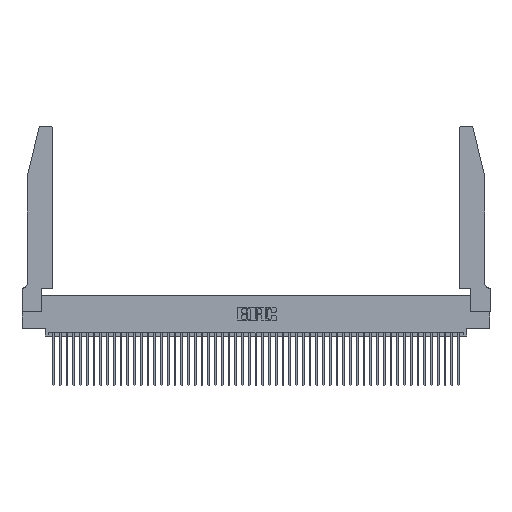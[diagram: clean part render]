
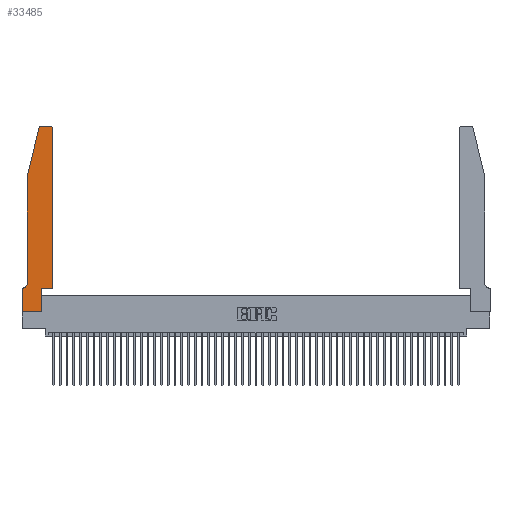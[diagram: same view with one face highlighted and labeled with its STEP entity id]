
A CAD part, top view. The second image highlights one B-rep face of the part: STEP entity #33485.
In plain terms, the highlighted planar face has unit normal (0, 0, 1).
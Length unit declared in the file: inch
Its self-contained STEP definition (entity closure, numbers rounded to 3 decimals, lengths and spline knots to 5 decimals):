
#647 = ORIENTED_EDGE ( 'NONE', *, *, #27246, .T. ) ;
#713 = LINE ( 'NONE', #17386, #20215 ) ;
#718 = CARTESIAN_POINT ( 'NONE',  ( 0.4505, 2.72, 0.37 ) ) ;
#2544 = EDGE_CURVE ( 'NONE', #25162, #24397, #713, .T. ) ;
#3590 = CARTESIAN_POINT ( 'NONE',  ( 0.0755, 2., 0.37 ) ) ;
#3707 = CARTESIAN_POINT ( 'NONE',  ( 0.2865, 0.35, 0.37 ) ) ;
#4420 = VECTOR ( 'NONE', #8207, 39.37008 ) ;
#6804 = ORIENTED_EDGE ( 'NONE', *, *, #12486, .T. ) ;
#7008 = DIRECTION ( 'NONE',  ( 0., 0., 1. ) ) ;
#7014 = DIRECTION ( 'NONE',  ( 0., 0., 1. ) ) ;
#7087 = VERTEX_POINT ( 'NONE', #14316 ) ;
#7631 = EDGE_LOOP ( 'NONE', ( #6804, #647, #19956, #20746, #41862, #13856, #21926, #33916, #32692, #13789, #16036, #45200 ) ) ;
#7732 = AXIS2_PLACEMENT_3D ( 'NONE', #43653, #20434, #47519 ) ;
#7896 = DIRECTION ( 'NONE',  ( 1., 0., 0. ) ) ;
#8207 = DIRECTION ( 'NONE',  ( -1., 0., 0. ) ) ;
#8855 = AXIS2_PLACEMENT_3D ( 'NONE', #42272, #19062, #46180 ) ;
#10037 = VERTEX_POINT ( 'NONE', #38490 ) ;
#12369 = VERTEX_POINT ( 'NONE', #46196 ) ;
#12486 = EDGE_CURVE ( 'NONE', #16111, #10037, #36589, .T. ) ;
#12656 = VECTOR ( 'NONE', #7896, 39.37008 ) ;
#12976 = EDGE_CURVE ( 'NONE', #24397, #7087, #18510, .T. ) ;
#13789 = ORIENTED_EDGE ( 'NONE', *, *, #38945, .T. ) ;
#13843 = DIRECTION ( 'NONE',  ( -1., 0., 0. ) ) ;
#13856 = ORIENTED_EDGE ( 'NONE', *, *, #46249, .T. ) ;
#13866 = LINE ( 'NONE', #15563, #12656 ) ;
#14316 = CARTESIAN_POINT ( 'NONE',  ( 0.2865, 0.35, 0.37 ) ) ;
#15222 = PLANE ( 'NONE',  #8855 ) ;
#15262 = CARTESIAN_POINT ( 'NONE',  ( 0.4505, 0.35, 0.37 ) ) ;
#15388 = CARTESIAN_POINT ( 'NONE',  ( 0., 0., 0.37 ) ) ;
#15453 = EDGE_CURVE ( 'NONE', #23237, #16111, #32829, .T. ) ;
#15563 = CARTESIAN_POINT ( 'NONE',  ( 0.4505, 0.35, 0.37 ) ) ;
#15775 = CARTESIAN_POINT ( 'NONE',  ( 0.25487, 2.72718, 0.37 ) ) ;
#16036 = ORIENTED_EDGE ( 'NONE', *, *, #18332, .T. ) ;
#16111 = VERTEX_POINT ( 'NONE', #19169 ) ;
#17232 = DIRECTION ( 'NONE',  ( 0., -1., 0. ) ) ;
#17386 = CARTESIAN_POINT ( 'NONE',  ( 0., 0., 0.37 ) ) ;
#17463 = VERTEX_POINT ( 'NONE', #41365 ) ;
#18332 = EDGE_CURVE ( 'NONE', #20852, #23237, #23528, .T. ) ;
#18510 = LINE ( 'NONE', #3707, #48184 ) ;
#19062 = DIRECTION ( 'NONE',  ( 0., 0., 1. ) ) ;
#19169 = CARTESIAN_POINT ( 'NONE',  ( 0.4205, 2.75, 0.37 ) ) ;
#19956 = ORIENTED_EDGE ( 'NONE', *, *, #48981, .T. ) ;
#20215 = VECTOR ( 'NONE', #44496, 39.37008 ) ;
#20434 = DIRECTION ( 'NONE',  ( 0., 0., -1. ) ) ;
#20746 = ORIENTED_EDGE ( 'NONE', *, *, #31628, .T. ) ;
#20852 = VERTEX_POINT ( 'NONE', #49442 ) ;
#21926 = ORIENTED_EDGE ( 'NONE', *, *, #24889, .T. ) ;
#23237 = VERTEX_POINT ( 'NONE', #718 ) ;
#23528 = LINE ( 'NONE', #15262, #44100 ) ;
#24397 = VERTEX_POINT ( 'NONE', #30204 ) ;
#24889 = EDGE_CURVE ( 'NONE', #26045, #25162, #47878, .T. ) ;
#25162 = VERTEX_POINT ( 'NONE', #15388 ) ;
#25265 = VECTOR ( 'NONE', #39976, 39.37008 ) ;
#26044 = LINE ( 'NONE', #3590, #33894 ) ;
#26045 = VERTEX_POINT ( 'NONE', #29202 ) ;
#26130 = VECTOR ( 'NONE', #17232, 39.37008 ) ;
#26546 = CIRCLE ( 'NONE', #36885, 0.03 ) ;
#27246 = EDGE_CURVE ( 'NONE', #10037, #40336, #26546, .T. ) ;
#28882 = VERTEX_POINT ( 'NONE', #28950 ) ;
#28950 = CARTESIAN_POINT ( 'NONE',  ( 0.0755, 2., 0.37 ) ) ;
#29202 = CARTESIAN_POINT ( 'NONE',  ( 0., 0.35, 0.37 ) ) ;
#29277 = CARTESIAN_POINT ( 'NONE',  ( 0.0755, 0.35, 0.37 ) ) ;
#30204 = CARTESIAN_POINT ( 'NONE',  ( 0.2865, 0., 0.37 ) ) ;
#30283 = CARTESIAN_POINT ( 'NONE',  ( 0.4205, 2.72, 0.37 ) ) ;
#30292 = CARTESIAN_POINT ( 'NONE',  ( 0.284, 2.72, 0.37 ) ) ;
#30936 = LINE ( 'NONE', #29277, #46584 ) ;
#31628 = EDGE_CURVE ( 'NONE', #28882, #17463, #26044, .T. ) ;
#32218 = CARTESIAN_POINT ( 'NONE',  ( 0.0755, 2., 0.37 ) ) ;
#32692 = ORIENTED_EDGE ( 'NONE', *, *, #12976, .T. ) ;
#32829 = CIRCLE ( 'NONE', #35489, 0.03 ) ;
#33485 = ADVANCED_FACE ( 'NONE', ( #45192 ), #15222, .T. ) ;
#33894 = VECTOR ( 'NONE', #50013, 39.37008 ) ;
#33916 = ORIENTED_EDGE ( 'NONE', *, *, #2544, .T. ) ;
#34160 = DIRECTION ( 'NONE',  ( 1., 0., 0. ) ) ;
#34165 = DIRECTION ( 'NONE',  ( 1., 0., 0. ) ) ;
#34785 = DIRECTION ( 'NONE',  ( 0., 1., 0. ) ) ;
#35314 = CARTESIAN_POINT ( 'NONE',  ( 0.2605, 2.75, 0.37 ) ) ;
#35489 = AXIS2_PLACEMENT_3D ( 'NONE', #30283, #7008, #34160 ) ;
#35512 = LINE ( 'NONE', #32218, #25265 ) ;
#36040 = CIRCLE ( 'NONE', #7732, 0.07 ) ;
#36589 = LINE ( 'NONE', #35314, #4420 ) ;
#36885 = AXIS2_PLACEMENT_3D ( 'NONE', #30292, #7014, #34165 ) ;
#38411 = DIRECTION ( 'NONE',  ( 0., 1., 0. ) ) ;
#38490 = CARTESIAN_POINT ( 'NONE',  ( 0.284, 2.75, 0.37 ) ) ;
#38945 = EDGE_CURVE ( 'NONE', #7087, #20852, #13866, .T. ) ;
#39976 = DIRECTION ( 'NONE',  ( -0.239, -0.971, 0. ) ) ;
#40336 = VERTEX_POINT ( 'NONE', #15775 ) ;
#40891 = EDGE_CURVE ( 'NONE', #17463, #12369, #36040, .T. ) ;
#41365 = CARTESIAN_POINT ( 'NONE',  ( 0.0755, 0.42, 0.37 ) ) ;
#41862 = ORIENTED_EDGE ( 'NONE', *, *, #40891, .T. ) ;
#42272 = CARTESIAN_POINT ( 'NONE',  ( 0., 0.35, 0.37 ) ) ;
#43653 = CARTESIAN_POINT ( 'NONE',  ( 0.0055, 0.42, 0.37 ) ) ;
#44100 = VECTOR ( 'NONE', #38411, 39.37008 ) ;
#44345 = CARTESIAN_POINT ( 'NONE',  ( 0., 0., 0.37 ) ) ;
#44496 = DIRECTION ( 'NONE',  ( 1., 0., 0. ) ) ;
#45192 = FACE_OUTER_BOUND ( 'NONE', #7631, .T. ) ;
#45200 = ORIENTED_EDGE ( 'NONE', *, *, #15453, .T. ) ;
#46180 = DIRECTION ( 'NONE',  ( 1., 0., 0. ) ) ;
#46196 = CARTESIAN_POINT ( 'NONE',  ( 0.0055, 0.35, 0.37 ) ) ;
#46249 = EDGE_CURVE ( 'NONE', #12369, #26045, #30936, .T. ) ;
#46584 = VECTOR ( 'NONE', #13843, 39.37008 ) ;
#47519 = DIRECTION ( 'NONE',  ( -1., 0., 0. ) ) ;
#47878 = LINE ( 'NONE', #44345, #26130 ) ;
#48184 = VECTOR ( 'NONE', #34785, 39.37008 ) ;
#48981 = EDGE_CURVE ( 'NONE', #40336, #28882, #35512, .T. ) ;
#49442 = CARTESIAN_POINT ( 'NONE',  ( 0.4505, 0.35, 0.37 ) ) ;
#50013 = DIRECTION ( 'NONE',  ( 0., -1., 0. ) ) ;
